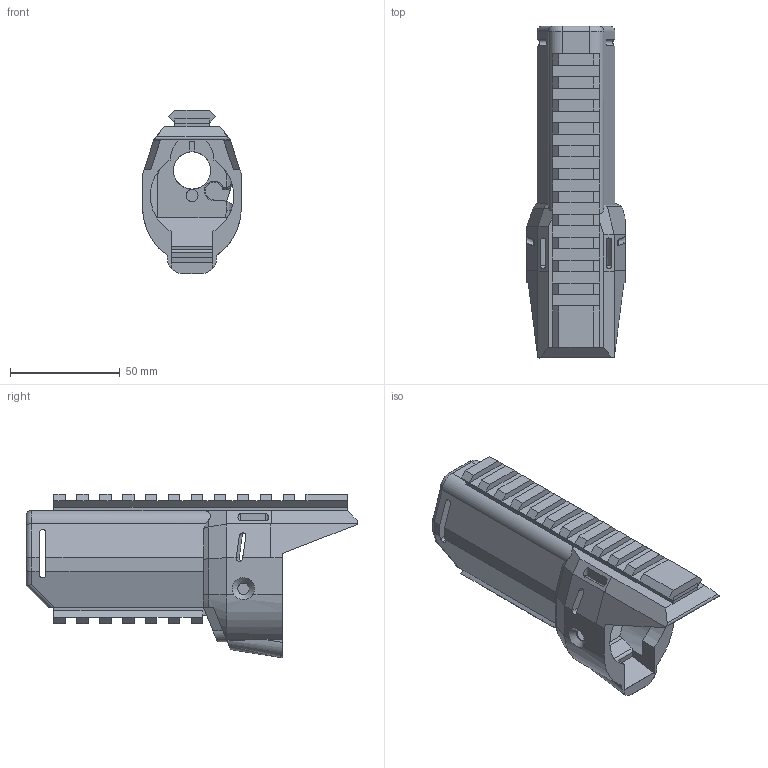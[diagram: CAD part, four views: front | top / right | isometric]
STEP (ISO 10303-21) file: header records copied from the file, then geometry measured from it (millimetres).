
FILE_DESCRIPTION(/* description */ (''),/* implementation_level */ '2;1');
FILE_NAME(/* name */ 'HRR PRA - 3.5 in Model v2.step',/* time_stamp */ '2020-04-20T22:02:16-04:00',/* author */ (''),/* organization */ (''),/* preprocessor_version */ 'ST-DEVELOPER v18.1',/* originating_system */ 'Autodesk Translation Framework v9.2.0.1227',/* authorisation */ '');
FILE_SCHEMA (('AUTOMOTIVE_DESIGN { 1 0 10303 214 3 1 1 }'));
Length unit declared in the file: inch
Products named in the file (2): HRR PRA - 3.5 in Model; Birdhead3.5
Assembly tree (1 placements, depth 2):
  HRR PRA - 3.5 in Model
    Birdhead3.5
Bounding box: 45 x 151.56 x 74.58 mm (x, y, z)
Volume: 145990.2 mm3; surface area: 52269 mm2
Topology: 3 solids, 3 shells, 366 faces, 1036 edges, 660 vertices
Faces by surface type: plane 299, cylinder 48, bspline 10, cone 6, torus 3
Full cylindrical faces by diameter (mm): 5.207 x1, 5.5 x1, 17 x2
Entity records: 11939 total; most frequent: CARTESIAN_POINT 2363, ORIENTED_EDGE 2072, DIRECTION 1886, EDGE_CURVE 1036, LINE 844, VECTOR 844, VERTEX_POINT 660, AXIS2_PLACEMENT_3D 521
